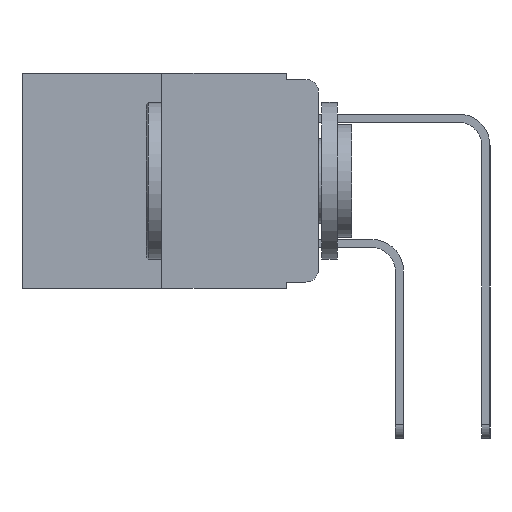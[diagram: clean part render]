
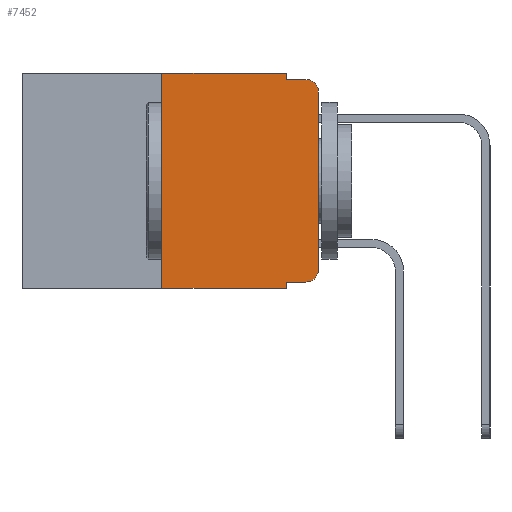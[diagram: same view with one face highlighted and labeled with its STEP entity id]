
A CAD part, left-side view. The second image highlights one B-rep face of the part: STEP entity #7452.
In plain terms, the highlighted planar face has unit normal (-1, 0, 0).
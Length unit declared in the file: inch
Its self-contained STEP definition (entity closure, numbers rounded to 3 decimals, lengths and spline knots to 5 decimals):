
#255 = ORIENTED_EDGE ( 'NONE', *, *, #3310, .T. ) ;
#554 = DIRECTION ( 'NONE',  ( 0., 0., -1. ) ) ;
#989 = FACE_OUTER_BOUND ( 'NONE', #12223, .T. ) ;
#1026 = CARTESIAN_POINT ( 'NONE',  ( 0., 0.051, -0.01 ) ) ;
#1188 = LINE ( 'NONE', #7988, #9767 ) ;
#1599 = LINE ( 'NONE', #11782, #3649 ) ;
#1731 = VECTOR ( 'NONE', #1907, 39.37008 ) ;
#1824 = VERTEX_POINT ( 'NONE', #1943 ) ;
#1855 = DIRECTION ( 'NONE',  ( 0., -1., 0. ) ) ;
#1907 = DIRECTION ( 'NONE',  ( 0., -1., 0. ) ) ;
#1943 = CARTESIAN_POINT ( 'NONE',  ( 0., 0.02, -0.333 ) ) ;
#1957 = LINE ( 'NONE', #2809, #10825 ) ;
#2225 = CARTESIAN_POINT ( 'NONE',  ( 0., 0., -0.313 ) ) ;
#2312 = EDGE_CURVE ( 'NONE', #1824, #8021, #10697, .T. ) ;
#2320 = VECTOR ( 'NONE', #15033, 39.37008 ) ;
#2586 = VERTEX_POINT ( 'NONE', #12743 ) ;
#2710 = AXIS2_PLACEMENT_3D ( 'NONE', #13257, #13150, #6342 ) ;
#2758 = DIRECTION ( 'NONE',  ( 0., 0., -1. ) ) ;
#2809 = CARTESIAN_POINT ( 'NONE',  ( 0., 0.051, 0. ) ) ;
#3008 = ORIENTED_EDGE ( 'NONE', *, *, #8534, .T. ) ;
#3101 = EDGE_CURVE ( 'NONE', #9355, #1824, #1599, .T. ) ;
#3165 = CARTESIAN_POINT ( 'NONE',  ( 0., 0.473, 0. ) ) ;
#3310 = EDGE_CURVE ( 'NONE', #3329, #2586, #13680, .T. ) ;
#3329 = VERTEX_POINT ( 'NONE', #5963 ) ;
#3598 = CIRCLE ( 'NONE', #13449, 0.02 ) ;
#3649 = VECTOR ( 'NONE', #7247, 39.37008 ) ;
#3869 = EDGE_CURVE ( 'NONE', #9355, #2586, #1957, .T. ) ;
#4064 = CARTESIAN_POINT ( 'NONE',  ( 0., 0.25, 0. ) ) ;
#4644 = EDGE_CURVE ( 'NONE', #3329, #5030, #1188, .T. ) ;
#4682 = PLANE ( 'NONE',  #11438 ) ;
#4931 = CARTESIAN_POINT ( 'NONE',  ( 0., 0.051, -0.01 ) ) ;
#5030 = VERTEX_POINT ( 'NONE', #4064 ) ;
#5367 = VECTOR ( 'NONE', #7368, 39.37008 ) ;
#5420 = EDGE_CURVE ( 'NONE', #11026, #6057, #11166, .T. ) ;
#5645 = DIRECTION ( 'NONE',  ( 0., 0., 1. ) ) ;
#5675 = ORIENTED_EDGE ( 'NONE', *, *, #2312, .T. ) ;
#5848 = ORIENTED_EDGE ( 'NONE', *, *, #7879, .F. ) ;
#5866 = CARTESIAN_POINT ( 'NONE',  ( 0., 0.473, 0. ) ) ;
#5963 = CARTESIAN_POINT ( 'NONE',  ( 0., 0.25, -0.343 ) ) ;
#6057 = VERTEX_POINT ( 'NONE', #1026 ) ;
#6218 = CARTESIAN_POINT ( 'NONE',  ( 0., 0., 0. ) ) ;
#6224 = EDGE_CURVE ( 'NONE', #6057, #8146, #12909, .T. ) ;
#6342 = DIRECTION ( 'NONE',  ( 0., 0., -1. ) ) ;
#7035 = DIRECTION ( 'NONE',  ( 0., 0., -1. ) ) ;
#7133 = CARTESIAN_POINT ( 'NONE',  ( 0., 0., -0.03 ) ) ;
#7247 = DIRECTION ( 'NONE',  ( 0., -1., 0. ) ) ;
#7261 = CARTESIAN_POINT ( 'NONE',  ( 0., 0.473, -0.343 ) ) ;
#7276 = VECTOR ( 'NONE', #1855, 39.37008 ) ;
#7368 = DIRECTION ( 'NONE',  ( 0., 0., 1. ) ) ;
#7452 = ADVANCED_FACE ( 'NONE', ( #989 ), #4682, .F. ) ;
#7625 = DIRECTION ( 'NONE',  ( -1., 0., 0. ) ) ;
#7776 = EDGE_CURVE ( 'NONE', #10972, #8146, #3598, .T. ) ;
#7879 = EDGE_CURVE ( 'NONE', #5030, #11026, #7949, .T. ) ;
#7949 = LINE ( 'NONE', #3165, #1731 ) ;
#7988 = CARTESIAN_POINT ( 'NONE',  ( 0., 0.25, 0. ) ) ;
#8021 = VERTEX_POINT ( 'NONE', #2225 ) ;
#8146 = VERTEX_POINT ( 'NONE', #9417 ) ;
#8534 = EDGE_CURVE ( 'NONE', #8021, #10972, #11129, .T. ) ;
#9355 = VERTEX_POINT ( 'NONE', #10154 ) ;
#9417 = CARTESIAN_POINT ( 'NONE',  ( 0., 0.02, -0.01 ) ) ;
#9442 = ORIENTED_EDGE ( 'NONE', *, *, #7776, .T. ) ;
#9767 = VECTOR ( 'NONE', #5645, 39.37008 ) ;
#9899 = VECTOR ( 'NONE', #13010, 39.37008 ) ;
#10154 = CARTESIAN_POINT ( 'NONE',  ( 0., 0.051, -0.333 ) ) ;
#10672 = CARTESIAN_POINT ( 'NONE',  ( 0., 0.051, 0. ) ) ;
#10697 = CIRCLE ( 'NONE', #2710, 0.02 ) ;
#10825 = VECTOR ( 'NONE', #2758, 39.37008 ) ;
#10972 = VERTEX_POINT ( 'NONE', #7133 ) ;
#11026 = VERTEX_POINT ( 'NONE', #10672 ) ;
#11129 = LINE ( 'NONE', #6218, #5367 ) ;
#11166 = LINE ( 'NONE', #13913, #2320 ) ;
#11218 = ORIENTED_EDGE ( 'NONE', *, *, #5420, .F. ) ;
#11438 = AXIS2_PLACEMENT_3D ( 'NONE', #5866, #13837, #7035 ) ;
#11782 = CARTESIAN_POINT ( 'NONE',  ( 0., 0.051, -0.333 ) ) ;
#12223 = EDGE_LOOP ( 'NONE', ( #3008, #9442, #13163, #11218, #5848, #13701, #255, #12658, #13370, #5675 ) ) ;
#12658 = ORIENTED_EDGE ( 'NONE', *, *, #3869, .F. ) ;
#12743 = CARTESIAN_POINT ( 'NONE',  ( 0., 0.051, -0.343 ) ) ;
#12909 = LINE ( 'NONE', #4931, #9899 ) ;
#13010 = DIRECTION ( 'NONE',  ( 0., -1., 0. ) ) ;
#13150 = DIRECTION ( 'NONE',  ( -1., 0., 0. ) ) ;
#13163 = ORIENTED_EDGE ( 'NONE', *, *, #6224, .F. ) ;
#13257 = CARTESIAN_POINT ( 'NONE',  ( 0., 0.02, -0.313 ) ) ;
#13370 = ORIENTED_EDGE ( 'NONE', *, *, #3101, .T. ) ;
#13449 = AXIS2_PLACEMENT_3D ( 'NONE', #14412, #7625, #554 ) ;
#13680 = LINE ( 'NONE', #7261, #7276 ) ;
#13701 = ORIENTED_EDGE ( 'NONE', *, *, #4644, .F. ) ;
#13837 = DIRECTION ( 'NONE',  ( 1., 0., 0. ) ) ;
#13913 = CARTESIAN_POINT ( 'NONE',  ( 0., 0.051, 0. ) ) ;
#14412 = CARTESIAN_POINT ( 'NONE',  ( 0., 0.02, -0.03 ) ) ;
#15033 = DIRECTION ( 'NONE',  ( 0., 0., -1. ) ) ;
